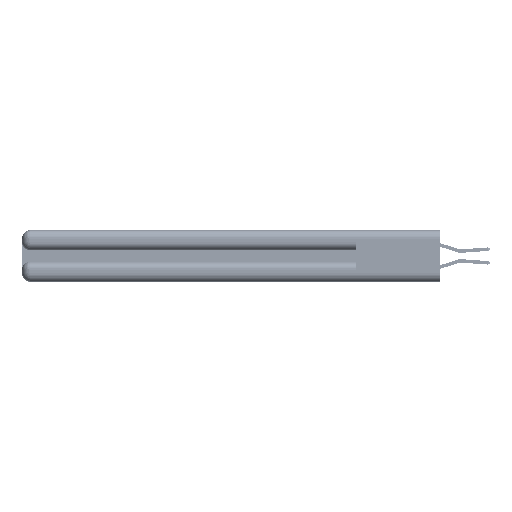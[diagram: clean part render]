
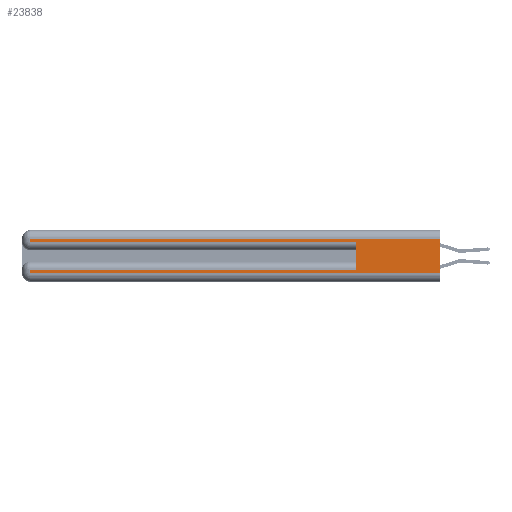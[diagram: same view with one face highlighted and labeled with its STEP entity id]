
A CAD part, left-side view. The second image highlights one B-rep face of the part: STEP entity #23838.
In plain terms, the highlighted planar face has unit normal (-1, 0, 0).
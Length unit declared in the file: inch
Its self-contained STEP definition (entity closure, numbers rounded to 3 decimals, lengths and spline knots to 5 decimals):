
#919 = ORIENTED_EDGE ( 'NONE', *, *, #12330, .T. ) ;
#2855 = DIRECTION ( 'NONE',  ( 0., -1., 0. ) ) ;
#3059 = VECTOR ( 'NONE', #32778, 39.37008 ) ;
#3325 = CARTESIAN_POINT ( 'NONE',  ( 0., 0., 0.085 ) ) ;
#3619 = CARTESIAN_POINT ( 'NONE',  ( 0., 0., 0.37 ) ) ;
#3745 = VERTEX_POINT ( 'NONE', #25023 ) ;
#4033 = VERTEX_POINT ( 'NONE', #31139 ) ;
#5777 = CARTESIAN_POINT ( 'NONE',  ( 0., 0., 0.06 ) ) ;
#6917 = ORIENTED_EDGE ( 'NONE', *, *, #25165, .T. ) ;
#7200 = CARTESIAN_POINT ( 'NONE',  ( 0., 0.6, 0.285 ) ) ;
#7228 = ORIENTED_EDGE ( 'NONE', *, *, #15648, .T. ) ;
#7755 = DIRECTION ( 'NONE',  ( 0., 0., -1. ) ) ;
#8067 = CARTESIAN_POINT ( 'NONE',  ( 0., 0., 0.31 ) ) ;
#8699 = CARTESIAN_POINT ( 'NONE',  ( 0., 2.94, 0.285 ) ) ;
#9020 = CARTESIAN_POINT ( 'NONE',  ( 0., 0., 0.06 ) ) ;
#9692 = VERTEX_POINT ( 'NONE', #8699 ) ;
#11217 = ORIENTED_EDGE ( 'NONE', *, *, #15660, .F. ) ;
#12041 = ORIENTED_EDGE ( 'NONE', *, *, #44495, .T. ) ;
#12050 = VERTEX_POINT ( 'NONE', #9020 ) ;
#12330 = EDGE_CURVE ( 'NONE', #50406, #17348, #26112, .T. ) ;
#12779 = VECTOR ( 'NONE', #27921, 39.37008 ) ;
#13985 = LINE ( 'NONE', #28631, #3059 ) ;
#15172 = VECTOR ( 'NONE', #33361, 39.37008 ) ;
#15648 = EDGE_CURVE ( 'NONE', #9692, #20672, #48412, .T. ) ;
#15660 = EDGE_CURVE ( 'NONE', #20802, #12050, #47143, .T. ) ;
#17216 = CARTESIAN_POINT ( 'NONE',  ( 0., 2.94, 0.06 ) ) ;
#17348 = VERTEX_POINT ( 'NONE', #17216 ) ;
#17719 = CARTESIAN_POINT ( 'NONE',  ( 0., 2.94, 0.37 ) ) ;
#18449 = CARTESIAN_POINT ( 'NONE',  ( 0., 0.6, 0.145 ) ) ;
#20672 = VERTEX_POINT ( 'NONE', #7200 ) ;
#20802 = VERTEX_POINT ( 'NONE', #8067 ) ;
#21857 = DIRECTION ( 'NONE',  ( 0., 0., -1. ) ) ;
#23499 = CARTESIAN_POINT ( 'NONE',  ( 0., 0., 0.37 ) ) ;
#23712 = LINE ( 'NONE', #3325, #12779 ) ;
#23838 = ADVANCED_FACE ( 'NONE', ( #52045 ), #28221, .F. ) ;
#24477 = LINE ( 'NONE', #18449, #31574 ) ;
#24960 = LINE ( 'NONE', #17719, #45544 ) ;
#25023 = CARTESIAN_POINT ( 'NONE',  ( 0., 0.6, 0.085 ) ) ;
#25165 = EDGE_CURVE ( 'NONE', #3745, #50406, #23712, .T. ) ;
#26112 = LINE ( 'NONE', #45209, #15172 ) ;
#26579 = VECTOR ( 'NONE', #2855, 39.37008 ) ;
#26720 = DIRECTION ( 'NONE',  ( 0., 0., 1. ) ) ;
#27921 = DIRECTION ( 'NONE',  ( 0., 1., 0. ) ) ;
#28221 = PLANE ( 'NONE',  #36887 ) ;
#28631 = CARTESIAN_POINT ( 'NONE',  ( 0., 0., 0.31 ) ) ;
#29211 = LINE ( 'NONE', #5777, #49772 ) ;
#29513 = CARTESIAN_POINT ( 'NONE',  ( 0., 2.94, 0.085 ) ) ;
#30114 = EDGE_LOOP ( 'NONE', ( #11217, #52181, #12041, #7228, #32977, #6917, #919, #51372 ) ) ;
#30583 = DIRECTION ( 'NONE',  ( 0., -1., 0. ) ) ;
#31139 = CARTESIAN_POINT ( 'NONE',  ( 0., 2.94, 0.31 ) ) ;
#31574 = VECTOR ( 'NONE', #26720, 39.37008 ) ;
#31600 = CARTESIAN_POINT ( 'NONE',  ( 0., 0., 0.285 ) ) ;
#32373 = DIRECTION ( 'NONE',  ( 1., 0., 0. ) ) ;
#32778 = DIRECTION ( 'NONE',  ( 0., 1., 0. ) ) ;
#32977 = ORIENTED_EDGE ( 'NONE', *, *, #43009, .F. ) ;
#33361 = DIRECTION ( 'NONE',  ( 0., 0., -1. ) ) ;
#36887 = AXIS2_PLACEMENT_3D ( 'NONE', #3619, #32373, #7755 ) ;
#36911 = EDGE_CURVE ( 'NONE', #17348, #12050, #29211, .T. ) ;
#37511 = VECTOR ( 'NONE', #43834, 39.37008 ) ;
#43009 = EDGE_CURVE ( 'NONE', #3745, #20672, #24477, .T. ) ;
#43834 = DIRECTION ( 'NONE',  ( 0., 0., -1. ) ) ;
#44495 = EDGE_CURVE ( 'NONE', #4033, #9692, #24960, .T. ) ;
#44926 = EDGE_CURVE ( 'NONE', #20802, #4033, #13985, .T. ) ;
#45209 = CARTESIAN_POINT ( 'NONE',  ( 0., 2.94, 0.37 ) ) ;
#45544 = VECTOR ( 'NONE', #21857, 39.37008 ) ;
#47143 = LINE ( 'NONE', #23499, #37511 ) ;
#48412 = LINE ( 'NONE', #31600, #26579 ) ;
#49772 = VECTOR ( 'NONE', #30583, 39.37008 ) ;
#50406 = VERTEX_POINT ( 'NONE', #29513 ) ;
#51372 = ORIENTED_EDGE ( 'NONE', *, *, #36911, .T. ) ;
#52045 = FACE_OUTER_BOUND ( 'NONE', #30114, .T. ) ;
#52181 = ORIENTED_EDGE ( 'NONE', *, *, #44926, .T. ) ;
